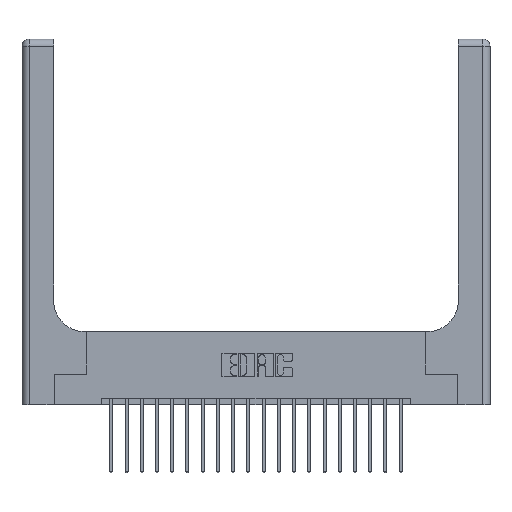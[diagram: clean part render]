
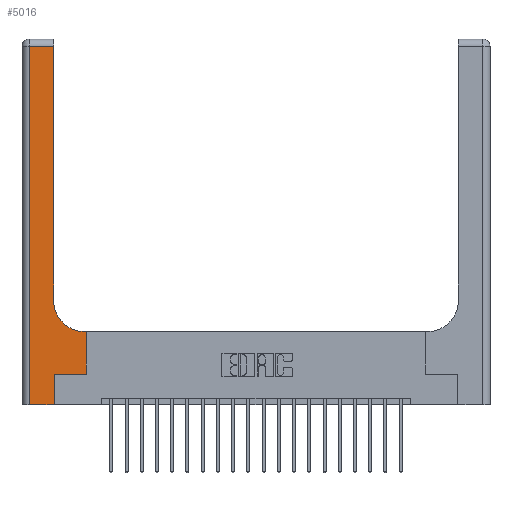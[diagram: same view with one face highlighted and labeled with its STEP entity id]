
A CAD part, top view. The second image highlights one B-rep face of the part: STEP entity #5016.
In plain terms, the highlighted planar face has unit normal (0, 0, 1).
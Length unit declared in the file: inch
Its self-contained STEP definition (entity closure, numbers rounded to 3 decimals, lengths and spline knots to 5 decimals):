
#879 = VERTEX_POINT ( 'NONE', #19738 ) ;
#1391 = EDGE_CURVE ( 'NONE', #5886, #3614, #13446, .T. ) ;
#1639 = LINE ( 'NONE', #7568, #9857 ) ;
#1955 = EDGE_CURVE ( 'NONE', #17776, #879, #1639, .T. ) ;
#2012 = CARTESIAN_POINT ( 'NONE',  ( 0.26, 0.85, 0.37 ) ) ;
#2097 = ORIENTED_EDGE ( 'NONE', *, *, #18264, .T. ) ;
#2115 = ORIENTED_EDGE ( 'NONE', *, *, #10053, .T. ) ;
#2410 = VERTEX_POINT ( 'NONE', #9659 ) ;
#3588 = LINE ( 'NONE', #18311, #11813 ) ;
#3614 = VERTEX_POINT ( 'NONE', #2012 ) ;
#4424 = LINE ( 'NONE', #4692, #8016 ) ;
#4455 = CARTESIAN_POINT ( 'NONE',  ( 0.265, 0.25, 0.37 ) ) ;
#4692 = CARTESIAN_POINT ( 'NONE',  ( 0., 2.94, 0.37 ) ) ;
#4780 = DIRECTION ( 'NONE',  ( 1., 0., 0. ) ) ;
#4816 = LINE ( 'NONE', #19334, #12516 ) ;
#5016 = ADVANCED_FACE ( 'NONE', ( #19980 ), #7714, .F. ) ;
#5125 = VECTOR ( 'NONE', #18603, 39.37008 ) ;
#5886 = VERTEX_POINT ( 'NONE', #14394 ) ;
#6005 = AXIS2_PLACEMENT_3D ( 'NONE', #19234, #9378, #11039 ) ;
#6546 = VERTEX_POINT ( 'NONE', #19095 ) ;
#6879 = LINE ( 'NONE', #8207, #9701 ) ;
#7568 = CARTESIAN_POINT ( 'NONE',  ( 0., 0., 0.37 ) ) ;
#7714 = PLANE ( 'NONE',  #6005 ) ;
#8016 = VECTOR ( 'NONE', #19451, 39.37008 ) ;
#8207 = CARTESIAN_POINT ( 'NONE',  ( 0.06, 3., 0.37 ) ) ;
#8619 = DIRECTION ( 'NONE',  ( 0., 0., -1. ) ) ;
#8759 = CARTESIAN_POINT ( 'NONE',  ( 0.51, 0.85, 0.37 ) ) ;
#8841 = ORIENTED_EDGE ( 'NONE', *, *, #18399, .T. ) ;
#9373 = ORIENTED_EDGE ( 'NONE', *, *, #1955, .T. ) ;
#9378 = DIRECTION ( 'NONE',  ( 0., 0., -1. ) ) ;
#9659 = CARTESIAN_POINT ( 'NONE',  ( 0.06, 2.94, 0.37 ) ) ;
#9665 = EDGE_CURVE ( 'NONE', #12512, #19608, #18002, .T. ) ;
#9695 = AXIS2_PLACEMENT_3D ( 'NONE', #8759, #8619, #13321 ) ;
#9701 = VECTOR ( 'NONE', #18076, 39.37008 ) ;
#9857 = VECTOR ( 'NONE', #12245, 39.37008 ) ;
#9892 = ORIENTED_EDGE ( 'NONE', *, *, #12107, .T. ) ;
#10053 = EDGE_CURVE ( 'NONE', #20286, #2410, #4424, .T. ) ;
#11039 = DIRECTION ( 'NONE',  ( -1., 0., 0. ) ) ;
#11164 = DIRECTION ( 'NONE',  ( 0., 1., 0. ) ) ;
#11498 = CARTESIAN_POINT ( 'NONE',  ( 0.528, 0.25, 0.37 ) ) ;
#11813 = VECTOR ( 'NONE', #19906, 39.37008 ) ;
#12107 = EDGE_CURVE ( 'NONE', #6546, #12512, #18689, .T. ) ;
#12245 = DIRECTION ( 'NONE',  ( 1., 0., 0. ) ) ;
#12512 = VERTEX_POINT ( 'NONE', #11498 ) ;
#12516 = VECTOR ( 'NONE', #20965, 39.37008 ) ;
#12880 = EDGE_CURVE ( 'NONE', #19608, #5886, #4816, .T. ) ;
#12930 = CARTESIAN_POINT ( 'NONE',  ( 0.06, 0., 0.37 ) ) ;
#12994 = EDGE_CURVE ( 'NONE', #2410, #17776, #6879, .T. ) ;
#13321 = DIRECTION ( 'NONE',  ( 1., 0., 0. ) ) ;
#13446 = CIRCLE ( 'NONE', #9695, 0.25 ) ;
#14394 = CARTESIAN_POINT ( 'NONE',  ( 0.51, 0.6, 0.37 ) ) ;
#14791 = ORIENTED_EDGE ( 'NONE', *, *, #1391, .T. ) ;
#15086 = LINE ( 'NONE', #17209, #5125 ) ;
#15593 = CARTESIAN_POINT ( 'NONE',  ( 0.528, 0.6, 0.37 ) ) ;
#15895 = ORIENTED_EDGE ( 'NONE', *, *, #12880, .T. ) ;
#17209 = CARTESIAN_POINT ( 'NONE',  ( 0.26, 3., 0.37 ) ) ;
#17776 = VERTEX_POINT ( 'NONE', #12930 ) ;
#18002 = LINE ( 'NONE', #19295, #18537 ) ;
#18076 = DIRECTION ( 'NONE',  ( 0., -1., 0. ) ) ;
#18264 = EDGE_CURVE ( 'NONE', #879, #6546, #3588, .T. ) ;
#18311 = CARTESIAN_POINT ( 'NONE',  ( 0.265, 0., 0.37 ) ) ;
#18399 = EDGE_CURVE ( 'NONE', #3614, #20286, #15086, .T. ) ;
#18459 = ORIENTED_EDGE ( 'NONE', *, *, #9665, .T. ) ;
#18537 = VECTOR ( 'NONE', #11164, 39.37008 ) ;
#18603 = DIRECTION ( 'NONE',  ( 0., 1., 0. ) ) ;
#18689 = LINE ( 'NONE', #4455, #20719 ) ;
#18821 = EDGE_LOOP ( 'NONE', ( #8841, #2115, #20663, #9373, #2097, #9892, #18459, #15895, #14791 ) ) ;
#19095 = CARTESIAN_POINT ( 'NONE',  ( 0.265, 0.25, 0.37 ) ) ;
#19177 = CARTESIAN_POINT ( 'NONE',  ( 0.26, 2.94, 0.37 ) ) ;
#19234 = CARTESIAN_POINT ( 'NONE',  ( 0., 3., 0.37 ) ) ;
#19295 = CARTESIAN_POINT ( 'NONE',  ( 0.528, 0.25, 0.37 ) ) ;
#19334 = CARTESIAN_POINT ( 'NONE',  ( 0.26, 0.6, 0.37 ) ) ;
#19451 = DIRECTION ( 'NONE',  ( -1., 0., 0. ) ) ;
#19608 = VERTEX_POINT ( 'NONE', #15593 ) ;
#19738 = CARTESIAN_POINT ( 'NONE',  ( 0.265, 0., 0.37 ) ) ;
#19906 = DIRECTION ( 'NONE',  ( 0., 1., 0. ) ) ;
#19980 = FACE_OUTER_BOUND ( 'NONE', #18821, .T. ) ;
#20286 = VERTEX_POINT ( 'NONE', #19177 ) ;
#20663 = ORIENTED_EDGE ( 'NONE', *, *, #12994, .T. ) ;
#20719 = VECTOR ( 'NONE', #4780, 39.37008 ) ;
#20965 = DIRECTION ( 'NONE',  ( -1., 0., 0. ) ) ;
